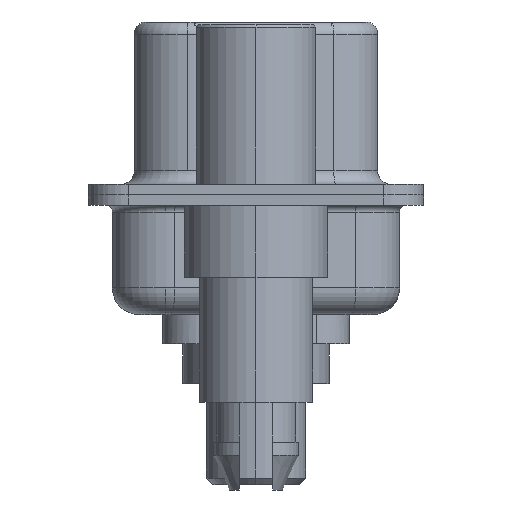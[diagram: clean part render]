
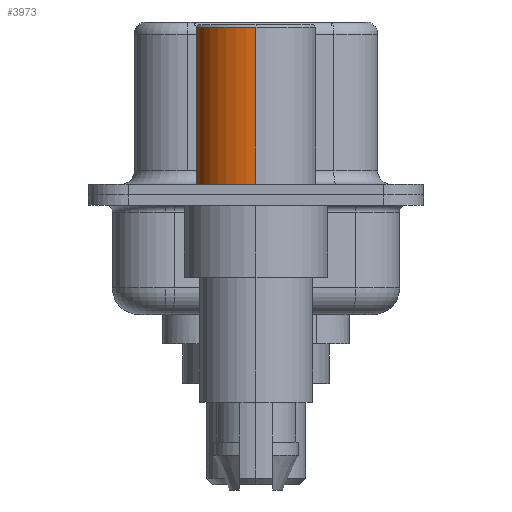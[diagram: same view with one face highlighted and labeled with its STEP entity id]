
A CAD part, left-side view. The second image highlights one B-rep face of the part: STEP entity #3973.
In plain terms, the highlighted cylindrical face has radius 2.25 mm (diameter 4.5 mm), a partial arc.
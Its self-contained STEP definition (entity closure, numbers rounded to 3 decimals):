
#4 = ORIENTED_EDGE ( 'NONE', *, *, #15356, .F. ) ;
#108 = CARTESIAN_POINT ( 'NONE',  ( 2.25, 0., 0.4 ) ) ;
#588 = LINE ( 'NONE', #11672, #2573 ) ;
#1144 = VERTEX_POINT ( 'NONE', #12172 ) ;
#1738 = DIRECTION ( 'NONE',  ( 1., 0., 0. ) ) ;
#2146 = EDGE_CURVE ( 'NONE', #12680, #1144, #13974, .T. ) ;
#2245 = VERTEX_POINT ( 'NONE', #5751 ) ;
#2386 = CARTESIAN_POINT ( 'NONE',  ( 0., 0., 0.4 ) ) ;
#2489 = ORIENTED_EDGE ( 'NONE', *, *, #2146, .T. ) ;
#2573 = VECTOR ( 'NONE', #12945, 1000. ) ;
#3693 = DIRECTION ( 'NONE',  ( 0., 0., 1. ) ) ;
#3973 = ADVANCED_FACE ( 'NONE', ( #16318 ), #7028, .T. ) ;
#4792 = AXIS2_PLACEMENT_3D ( 'NONE', #2386, #3693, #12661 ) ;
#4909 = DIRECTION ( 'NONE',  ( 1., 0., 0. ) ) ;
#5751 = CARTESIAN_POINT ( 'NONE',  ( 2.25, 0., 6.3 ) ) ;
#5886 = EDGE_LOOP ( 'NONE', ( #2489, #6470, #4, #12849 ) ) ;
#6470 = ORIENTED_EDGE ( 'NONE', *, *, #6822, .T. ) ;
#6691 = DIRECTION ( 'NONE',  ( 0., 0., 1. ) ) ;
#6822 = EDGE_CURVE ( 'NONE', #1144, #6988, #9307, .T. ) ;
#6988 = VERTEX_POINT ( 'NONE', #10595 ) ;
#7028 = CYLINDRICAL_SURFACE ( 'NONE', #9046, 2.25 ) ;
#7433 = AXIS2_PLACEMENT_3D ( 'NONE', #13091, #6691, #1738 ) ;
#9046 = AXIS2_PLACEMENT_3D ( 'NONE', #12490, #9878, #4909 ) ;
#9193 = EDGE_CURVE ( 'NONE', #12680, #2245, #588, .T. ) ;
#9307 = LINE ( 'NONE', #15039, #13857 ) ;
#9878 = DIRECTION ( 'NONE',  ( 0., 0., 1. ) ) ;
#10595 = CARTESIAN_POINT ( 'NONE',  ( -2.25, 0., 6.3 ) ) ;
#11635 = CIRCLE ( 'NONE', #7433, 2.25 ) ;
#11672 = CARTESIAN_POINT ( 'NONE',  ( 2.25, 0., 0.581 ) ) ;
#12172 = CARTESIAN_POINT ( 'NONE',  ( -2.25, 0., 0.4 ) ) ;
#12490 = CARTESIAN_POINT ( 'NONE',  ( 0., 0., 0.581 ) ) ;
#12651 = DIRECTION ( 'NONE',  ( 0., 0., 1. ) ) ;
#12661 = DIRECTION ( 'NONE',  ( 1., 0., 0. ) ) ;
#12680 = VERTEX_POINT ( 'NONE', #108 ) ;
#12849 = ORIENTED_EDGE ( 'NONE', *, *, #9193, .F. ) ;
#12945 = DIRECTION ( 'NONE',  ( 0., 0., 1. ) ) ;
#13091 = CARTESIAN_POINT ( 'NONE',  ( 0., 0., 6.3 ) ) ;
#13857 = VECTOR ( 'NONE', #12651, 1000. ) ;
#13974 = CIRCLE ( 'NONE', #4792, 2.25 ) ;
#15039 = CARTESIAN_POINT ( 'NONE',  ( -2.25, 0., 0.581 ) ) ;
#15356 = EDGE_CURVE ( 'NONE', #2245, #6988, #11635, .T. ) ;
#16318 = FACE_OUTER_BOUND ( 'NONE', #5886, .T. ) ;
